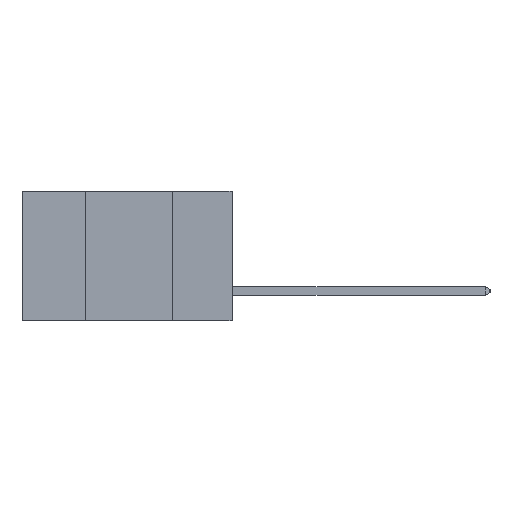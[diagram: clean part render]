
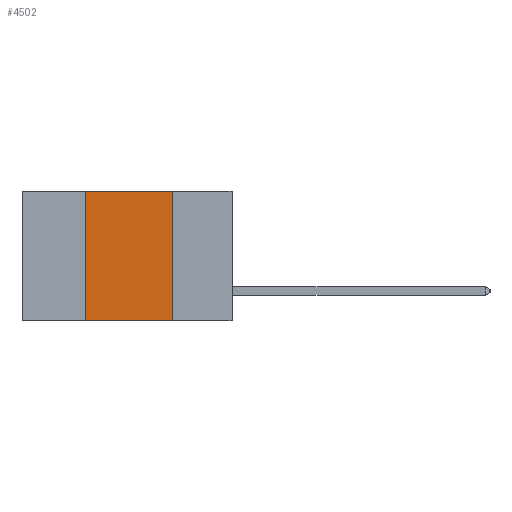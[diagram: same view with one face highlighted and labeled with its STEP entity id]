
A CAD part, left-side view. The second image highlights one B-rep face of the part: STEP entity #4502.
In plain terms, the highlighted planar face has unit normal (-1, 0, 0).
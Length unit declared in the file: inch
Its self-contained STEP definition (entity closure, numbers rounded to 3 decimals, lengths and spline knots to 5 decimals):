
#147 = VERTEX_POINT ( 'NONE', #16684 ) ;
#480 = EDGE_CURVE ( 'NONE', #147, #9584, #14003, .T. ) ;
#620 = EDGE_LOOP ( 'NONE', ( #12958, #13168, #12285, #12307 ) ) ;
#882 = VECTOR ( 'NONE', #14640, 39.37008 ) ;
#1008 = VECTOR ( 'NONE', #8230, 39.37008 ) ;
#2256 = CARTESIAN_POINT ( 'NONE',  ( 0., 0.6, -0.37 ) ) ;
#2594 = LINE ( 'NONE', #2256, #10941 ) ;
#4502 = ADVANCED_FACE ( 'NONE', ( #16371 ), #4642, .F. ) ;
#4561 = DIRECTION ( 'NONE',  ( 1., 0., 0. ) ) ;
#4642 = PLANE ( 'NONE',  #17271 ) ;
#4709 = DIRECTION ( 'NONE',  ( 0., 0., -1. ) ) ;
#4907 = CARTESIAN_POINT ( 'NONE',  ( 0., 0.6, 0. ) ) ;
#5563 = LINE ( 'NONE', #14550, #1008 ) ;
#6409 = VERTEX_POINT ( 'NONE', #9695 ) ;
#7177 = EDGE_CURVE ( 'NONE', #6409, #9971, #19046, .T. ) ;
#7285 = CARTESIAN_POINT ( 'NONE',  ( 0., 0.17, 0. ) ) ;
#7585 = EDGE_CURVE ( 'NONE', #9584, #6409, #5563, .T. ) ;
#8230 = DIRECTION ( 'NONE',  ( 0., -1., 0. ) ) ;
#8607 = CARTESIAN_POINT ( 'NONE',  ( 0., 0.17, -0.37 ) ) ;
#8901 = DIRECTION ( 'NONE',  ( 0., -1., 0. ) ) ;
#9584 = VERTEX_POINT ( 'NONE', #12005 ) ;
#9695 = CARTESIAN_POINT ( 'NONE',  ( 0., 0.17, 0. ) ) ;
#9971 = VERTEX_POINT ( 'NONE', #8607 ) ;
#10941 = VECTOR ( 'NONE', #8901, 39.37008 ) ;
#12005 = CARTESIAN_POINT ( 'NONE',  ( 0., 0.42, 0. ) ) ;
#12285 = ORIENTED_EDGE ( 'NONE', *, *, #480, .F. ) ;
#12307 = ORIENTED_EDGE ( 'NONE', *, *, #15271, .T. ) ;
#12958 = ORIENTED_EDGE ( 'NONE', *, *, #7177, .F. ) ;
#13168 = ORIENTED_EDGE ( 'NONE', *, *, #7585, .F. ) ;
#14003 = LINE ( 'NONE', #14845, #882 ) ;
#14550 = CARTESIAN_POINT ( 'NONE',  ( 0., 0.6, 0. ) ) ;
#14640 = DIRECTION ( 'NONE',  ( 0., 0., 1. ) ) ;
#14845 = CARTESIAN_POINT ( 'NONE',  ( 0., 0.42, 0. ) ) ;
#15271 = EDGE_CURVE ( 'NONE', #147, #9971, #2594, .T. ) ;
#16371 = FACE_OUTER_BOUND ( 'NONE', #620, .T. ) ;
#16684 = CARTESIAN_POINT ( 'NONE',  ( 0., 0.42, -0.37 ) ) ;
#17271 = AXIS2_PLACEMENT_3D ( 'NONE', #4907, #4561, #4709 ) ;
#18179 = DIRECTION ( 'NONE',  ( 0., 0., -1. ) ) ;
#19046 = LINE ( 'NONE', #7285, #19509 ) ;
#19509 = VECTOR ( 'NONE', #18179, 39.37008 ) ;
